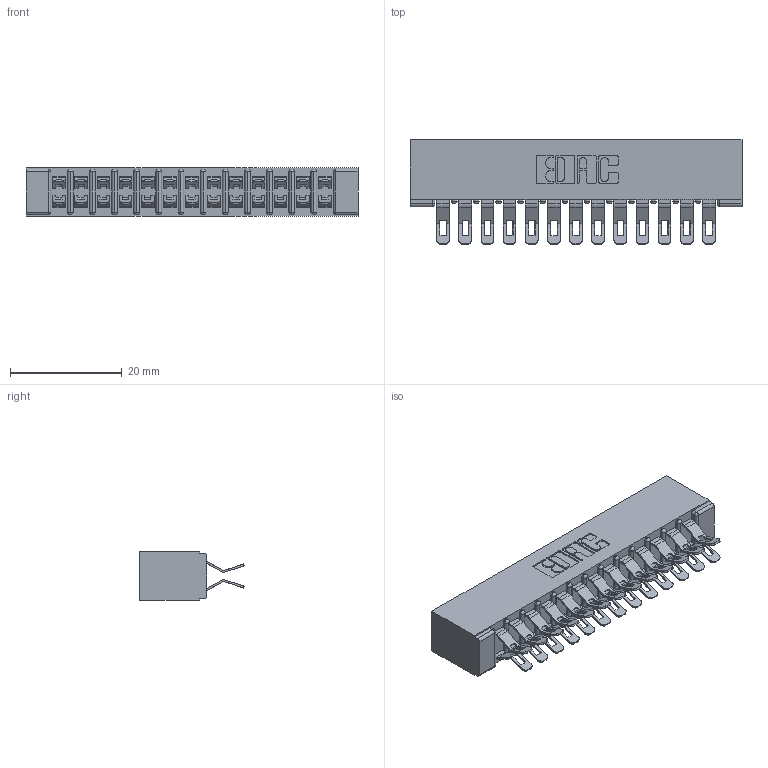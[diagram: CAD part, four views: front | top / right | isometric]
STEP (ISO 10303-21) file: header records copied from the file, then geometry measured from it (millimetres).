
FILE_DESCRIPTION (( 'STEP AP203' ), '1' );
FILE_NAME ('357-026-455-201.STEP', '2020-10-03T02:42:52', ( '' ), ( '' ), 'SwSTEP 2.0', 'SolidWorks 2020', '' );
FILE_SCHEMA (( 'CONFIG_CONTROL_DESIGN' ));
Length unit declared in the file: inch
Products named in the file (3): 357-026-455-201; 307 Part_No Mounting Lugs; 307-290-001_555
Assembly tree (27 placements, depth 2):
  357-026-455-201
    307 Part_No Mounting Lugs
    307-290-001_555  x26
Bounding box: 59.39 x 18.75 x 8.71 mm (x, y, z)
Volume: 4196 mm3; surface area: 7840.4 mm2
Topology: 27 solids, 27 shells, 1710 faces, 5005 edges, 3262 vertices
Faces by surface type: plane 950, cylinder 732, sphere 28
Entity records: 15395 total; most frequent: CARTESIAN_POINT 2529, ORIENTED_EDGE 2504, DIRECTION 2496, EDGE_CURVE 1252, VECTOR 938, LINE 938, VERTEX_POINT 812, AXIS2_PLACEMENT_3D 779
